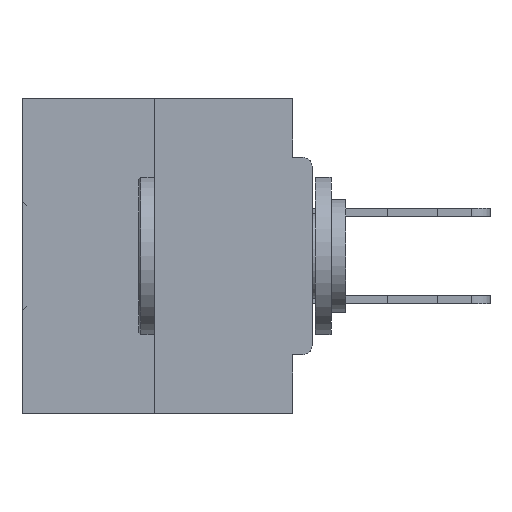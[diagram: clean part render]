
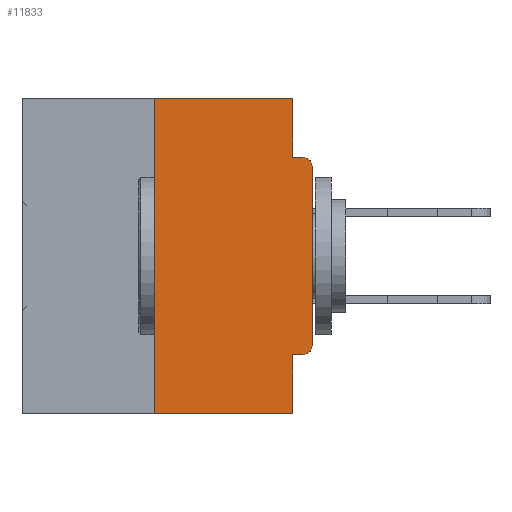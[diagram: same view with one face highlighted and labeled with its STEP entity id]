
A CAD part, left-side view. The second image highlights one B-rep face of the part: STEP entity #11833.
In plain terms, the highlighted planar face has unit normal (-1, 0, 0).
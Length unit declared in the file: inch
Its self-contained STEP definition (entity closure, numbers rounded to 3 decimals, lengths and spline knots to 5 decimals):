
#1649 = VERTEX_POINT ( 'NONE', #38801 ) ;
#1950 = DIRECTION ( 'NONE',  ( -1., 0., 0. ) ) ;
#3013 = VERTEX_POINT ( 'NONE', #34790 ) ;
#3372 = LINE ( 'NONE', #34036, #5039 ) ;
#3608 = EDGE_CURVE ( 'NONE', #26213, #29757, #46154, .T. ) ;
#5039 = VECTOR ( 'NONE', #44564, 39.37008 ) ;
#5180 = AXIS2_PLACEMENT_3D ( 'NONE', #8848, #1950, #19511 ) ;
#6008 = EDGE_CURVE ( 'NONE', #6956, #14404, #6069, .T. ) ;
#6069 = LINE ( 'NONE', #32456, #42038 ) ;
#6836 = VECTOR ( 'NONE', #39005, 39.37008 ) ;
#6956 = VERTEX_POINT ( 'NONE', #31086 ) ;
#7804 = ORIENTED_EDGE ( 'NONE', *, *, #36283, .F. ) ;
#7884 = ORIENTED_EDGE ( 'NONE', *, *, #10372, .F. ) ;
#8848 = CARTESIAN_POINT ( 'NONE',  ( 0., 0.015, -0.3915 ) ) ;
#9805 = VERTEX_POINT ( 'NONE', #35760 ) ;
#9809 = DIRECTION ( 'NONE',  ( -1., 0., 0. ) ) ;
#10372 = EDGE_CURVE ( 'NONE', #1649, #44737, #28695, .T. ) ;
#10980 = ORIENTED_EDGE ( 'NONE', *, *, #21836, .F. ) ;
#11833 = ADVANCED_FACE ( 'NONE', ( #46074 ), #38818, .F. ) ;
#13867 = CARTESIAN_POINT ( 'NONE',  ( 0., 0., -0.3915 ) ) ;
#14065 = CARTESIAN_POINT ( 'NONE',  ( 0., 0.46, 0. ) ) ;
#14111 = CARTESIAN_POINT ( 'NONE',  ( 0., 0., -0.4065 ) ) ;
#14404 = VERTEX_POINT ( 'NONE', #36071 ) ;
#15913 = LINE ( 'NONE', #35689, #41772 ) ;
#16006 = VERTEX_POINT ( 'NONE', #42192 ) ;
#17307 = DIRECTION ( 'NONE',  ( 1., 0., 0. ) ) ;
#18196 = DIRECTION ( 'NONE',  ( 0., -1., 0. ) ) ;
#18494 = ORIENTED_EDGE ( 'NONE', *, *, #3608, .T. ) ;
#19511 = DIRECTION ( 'NONE',  ( 0., 0., -1. ) ) ;
#19530 = DIRECTION ( 'NONE',  ( 0., 1., 0. ) ) ;
#20476 = CARTESIAN_POINT ( 'NONE',  ( 0., 0.015, -0.1085 ) ) ;
#21212 = CARTESIAN_POINT ( 'NONE',  ( 0., 0.46, 0. ) ) ;
#21836 = EDGE_CURVE ( 'NONE', #9805, #1649, #22293, .T. ) ;
#22293 = LINE ( 'NONE', #37615, #36896 ) ;
#22624 = LINE ( 'NONE', #34171, #34436 ) ;
#22769 = EDGE_CURVE ( 'NONE', #44737, #6956, #15913, .T. ) ;
#24835 = DIRECTION ( 'NONE',  ( 0., 0., -1. ) ) ;
#25022 = DIRECTION ( 'NONE',  ( 0., 0., -1. ) ) ;
#26213 = VERTEX_POINT ( 'NONE', #41094 ) ;
#26214 = AXIS2_PLACEMENT_3D ( 'NONE', #20476, #9809, #45470 ) ;
#28001 = DIRECTION ( 'NONE',  ( 0., -1., 0. ) ) ;
#28008 = EDGE_LOOP ( 'NONE', ( #7884, #10980, #43277, #45201, #7804, #18494, #45399, #45873, #29544, #32233 ) ) ;
#28115 = CARTESIAN_POINT ( 'NONE',  ( 0., 0.46, -0.5 ) ) ;
#28695 = LINE ( 'NONE', #14065, #34939 ) ;
#29544 = ORIENTED_EDGE ( 'NONE', *, *, #6008, .F. ) ;
#29757 = VERTEX_POINT ( 'NONE', #13867 ) ;
#31086 = CARTESIAN_POINT ( 'NONE',  ( 0., 0.031, -0.0935 ) ) ;
#32233 = ORIENTED_EDGE ( 'NONE', *, *, #22769, .F. ) ;
#32456 = CARTESIAN_POINT ( 'NONE',  ( 0., 0., -0.0935 ) ) ;
#33451 = EDGE_CURVE ( 'NONE', #16006, #14404, #44654, .T. ) ;
#33843 = DIRECTION ( 'NONE',  ( 0., 0., -1. ) ) ;
#34036 = CARTESIAN_POINT ( 'NONE',  ( 0., 0., 0. ) ) ;
#34171 = CARTESIAN_POINT ( 'NONE',  ( 0., 0.031, -0.5 ) ) ;
#34436 = VECTOR ( 'NONE', #33843, 39.37008 ) ;
#34790 = CARTESIAN_POINT ( 'NONE',  ( 0., 0.031, -0.4065 ) ) ;
#34939 = VECTOR ( 'NONE', #28001, 39.37008 ) ;
#35689 = CARTESIAN_POINT ( 'NONE',  ( 0., 0.031, 0. ) ) ;
#35760 = CARTESIAN_POINT ( 'NONE',  ( 0., 0.25, -0.5 ) ) ;
#35891 = EDGE_CURVE ( 'NONE', #3013, #44929, #22624, .T. ) ;
#36071 = CARTESIAN_POINT ( 'NONE',  ( 0., 0.015, -0.0935 ) ) ;
#36090 = VECTOR ( 'NONE', #19530, 39.37008 ) ;
#36283 = EDGE_CURVE ( 'NONE', #26213, #3013, #45712, .T. ) ;
#36896 = VECTOR ( 'NONE', #45000, 39.37008 ) ;
#36954 = CARTESIAN_POINT ( 'NONE',  ( 0., 0.031, -0.5 ) ) ;
#37615 = CARTESIAN_POINT ( 'NONE',  ( 0., 0.25, 0. ) ) ;
#38801 = CARTESIAN_POINT ( 'NONE',  ( 0., 0.25, 0. ) ) ;
#38818 = PLANE ( 'NONE',  #44965 ) ;
#39005 = DIRECTION ( 'NONE',  ( 0., -1., 0. ) ) ;
#41094 = CARTESIAN_POINT ( 'NONE',  ( 0., 0.015, -0.4065 ) ) ;
#41772 = VECTOR ( 'NONE', #25022, 39.37008 ) ;
#41856 = EDGE_CURVE ( 'NONE', #9805, #44929, #44464, .T. ) ;
#42038 = VECTOR ( 'NONE', #18196, 39.37008 ) ;
#42192 = CARTESIAN_POINT ( 'NONE',  ( 0., 0., -0.1085 ) ) ;
#42879 = EDGE_CURVE ( 'NONE', #29757, #16006, #3372, .T. ) ;
#43109 = CARTESIAN_POINT ( 'NONE',  ( 0., 0.031, 0. ) ) ;
#43277 = ORIENTED_EDGE ( 'NONE', *, *, #41856, .T. ) ;
#44464 = LINE ( 'NONE', #28115, #6836 ) ;
#44564 = DIRECTION ( 'NONE',  ( 0., 0., 1. ) ) ;
#44654 = CIRCLE ( 'NONE', #26214, 0.015 ) ;
#44737 = VERTEX_POINT ( 'NONE', #43109 ) ;
#44929 = VERTEX_POINT ( 'NONE', #36954 ) ;
#44965 = AXIS2_PLACEMENT_3D ( 'NONE', #21212, #17307, #24835 ) ;
#45000 = DIRECTION ( 'NONE',  ( 0., 0., 1. ) ) ;
#45201 = ORIENTED_EDGE ( 'NONE', *, *, #35891, .F. ) ;
#45399 = ORIENTED_EDGE ( 'NONE', *, *, #42879, .T. ) ;
#45470 = DIRECTION ( 'NONE',  ( 0., 0., -1. ) ) ;
#45712 = LINE ( 'NONE', #14111, #36090 ) ;
#45873 = ORIENTED_EDGE ( 'NONE', *, *, #33451, .T. ) ;
#46074 = FACE_OUTER_BOUND ( 'NONE', #28008, .T. ) ;
#46154 = CIRCLE ( 'NONE', #5180, 0.015 ) ;
